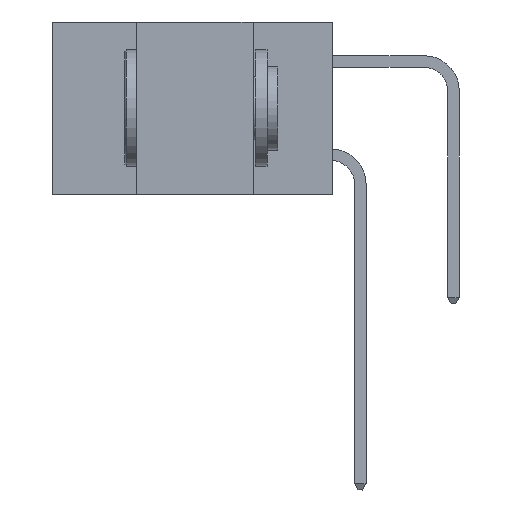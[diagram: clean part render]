
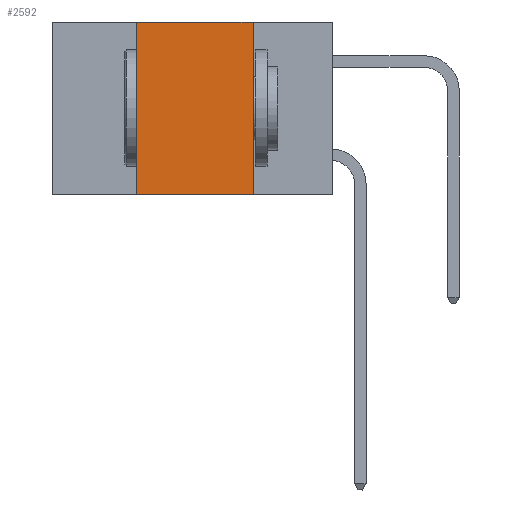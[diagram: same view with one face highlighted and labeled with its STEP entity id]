
A CAD part, left-side view. The second image highlights one B-rep face of the part: STEP entity #2592.
In plain terms, the highlighted planar face has unit normal (-1, 0, 0).
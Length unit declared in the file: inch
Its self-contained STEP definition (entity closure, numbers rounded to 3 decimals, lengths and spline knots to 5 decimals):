
#1469 = CARTESIAN_POINT ( 'NONE',  ( 0., 0.42, -0.37 ) ) ;
#1680 = VERTEX_POINT ( 'NONE', #1684 ) ;
#1684 = CARTESIAN_POINT ( 'NONE',  ( 0., 0.17, 0. ) ) ;
#2392 = VECTOR ( 'NONE', #5334, 39.37008 ) ;
#2592 = ADVANCED_FACE ( 'NONE', ( #3485 ), #15474, .F. ) ;
#3485 = FACE_OUTER_BOUND ( 'NONE', #21702, .T. ) ;
#4477 = DIRECTION ( 'NONE',  ( 0., -1., 0. ) ) ;
#4729 = DIRECTION ( 'NONE',  ( 0., 0., -1. ) ) ;
#5221 = DIRECTION ( 'NONE',  ( 0., 0., -1. ) ) ;
#5289 = CARTESIAN_POINT ( 'NONE',  ( 0., 0.17, -0.37 ) ) ;
#5334 = DIRECTION ( 'NONE',  ( 0., 0., 1. ) ) ;
#5559 = CARTESIAN_POINT ( 'NONE',  ( 0., 0.42, -0.37 ) ) ;
#5662 = AXIS2_PLACEMENT_3D ( 'NONE', #10572, #22535, #5221 ) ;
#6323 = CARTESIAN_POINT ( 'NONE',  ( 0., 0.6, 0. ) ) ;
#6651 = CARTESIAN_POINT ( 'NONE',  ( 0., 0.6, -0.37 ) ) ;
#7023 = EDGE_CURVE ( 'NONE', #16700, #1680, #8384, .T. ) ;
#7155 = VECTOR ( 'NONE', #4477, 39.37008 ) ;
#7986 = EDGE_CURVE ( 'NONE', #15202, #13894, #17238, .T. ) ;
#8234 = VECTOR ( 'NONE', #22234, 39.37008 ) ;
#8384 = LINE ( 'NONE', #6323, #7155 ) ;
#9068 = ORIENTED_EDGE ( 'NONE', *, *, #19107, .F. ) ;
#10572 = CARTESIAN_POINT ( 'NONE',  ( 0., 0.6, 0. ) ) ;
#10855 = EDGE_CURVE ( 'NONE', #1680, #13894, #18780, .T. ) ;
#13894 = VERTEX_POINT ( 'NONE', #5289 ) ;
#14695 = ORIENTED_EDGE ( 'NONE', *, *, #10855, .F. ) ;
#15202 = VERTEX_POINT ( 'NONE', #1469 ) ;
#15474 = PLANE ( 'NONE',  #5662 ) ;
#16700 = VERTEX_POINT ( 'NONE', #22469 ) ;
#17238 = LINE ( 'NONE', #6651, #8234 ) ;
#18780 = LINE ( 'NONE', #20425, #22818 ) ;
#18990 = ORIENTED_EDGE ( 'NONE', *, *, #7023, .F. ) ;
#19107 = EDGE_CURVE ( 'NONE', #15202, #16700, #19397, .T. ) ;
#19397 = LINE ( 'NONE', #5559, #2392 ) ;
#19678 = ORIENTED_EDGE ( 'NONE', *, *, #7986, .T. ) ;
#20425 = CARTESIAN_POINT ( 'NONE',  ( 0., 0.17, -0.37 ) ) ;
#21702 = EDGE_LOOP ( 'NONE', ( #14695, #18990, #9068, #19678 ) ) ;
#22234 = DIRECTION ( 'NONE',  ( 0., -1., 0. ) ) ;
#22469 = CARTESIAN_POINT ( 'NONE',  ( 0., 0.42, 0. ) ) ;
#22535 = DIRECTION ( 'NONE',  ( 1., 0., 0. ) ) ;
#22818 = VECTOR ( 'NONE', #4729, 39.37008 ) ;
